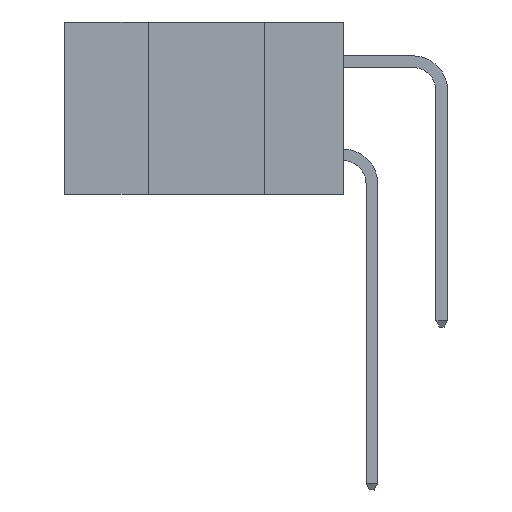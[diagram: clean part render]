
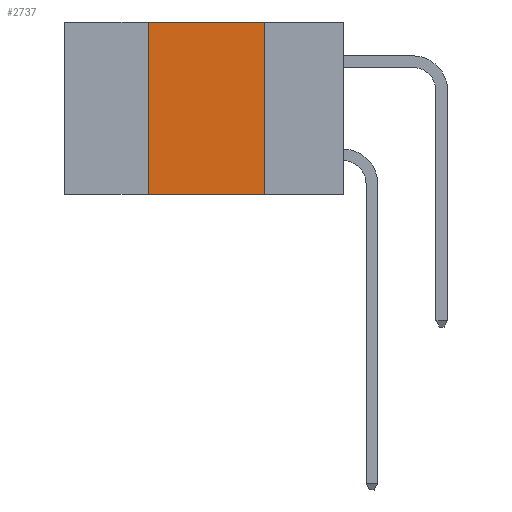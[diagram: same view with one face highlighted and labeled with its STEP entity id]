
A CAD part, left-side view. The second image highlights one B-rep face of the part: STEP entity #2737.
In plain terms, the highlighted planar face has unit normal (-1, 0, 0).
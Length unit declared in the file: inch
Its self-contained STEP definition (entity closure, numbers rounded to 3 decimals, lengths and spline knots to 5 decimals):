
#382 = DIRECTION ( 'NONE',  ( 0., -1., 0. ) ) ;
#444 = CARTESIAN_POINT ( 'NONE',  ( 0., 0.42, 0. ) ) ;
#821 = DIRECTION ( 'NONE',  ( 0., 0., 1. ) ) ;
#986 = CARTESIAN_POINT ( 'NONE',  ( 0., 0.42, -0.37 ) ) ;
#1899 = DIRECTION ( 'NONE',  ( 0., 0., -1. ) ) ;
#2342 = CARTESIAN_POINT ( 'NONE',  ( 0., 0.42, 0. ) ) ;
#2737 = ADVANCED_FACE ( 'NONE', ( #7547 ), #6748, .F. ) ;
#3230 = LINE ( 'NONE', #13689, #19517 ) ;
#4160 = CARTESIAN_POINT ( 'NONE',  ( 0., 0.6, 0. ) ) ;
#5080 = CARTESIAN_POINT ( 'NONE',  ( 0., 0.6, 0. ) ) ;
#5134 = VECTOR ( 'NONE', #821, 39.37008 ) ;
#5512 = LINE ( 'NONE', #9386, #15669 ) ;
#6301 = CARTESIAN_POINT ( 'NONE',  ( 0., 0.17, -0.37 ) ) ;
#6748 = PLANE ( 'NONE',  #14610 ) ;
#6756 = EDGE_CURVE ( 'NONE', #20666, #8106, #7747, .T. ) ;
#7547 = FACE_OUTER_BOUND ( 'NONE', #16509, .T. ) ;
#7600 = VECTOR ( 'NONE', #19569, 39.37008 ) ;
#7747 = LINE ( 'NONE', #2342, #5134 ) ;
#8106 = VERTEX_POINT ( 'NONE', #444 ) ;
#8134 = EDGE_CURVE ( 'NONE', #20666, #9131, #3230, .T. ) ;
#8920 = EDGE_CURVE ( 'NONE', #16882, #9131, #5512, .T. ) ;
#9131 = VERTEX_POINT ( 'NONE', #6301 ) ;
#9386 = CARTESIAN_POINT ( 'NONE',  ( 0., 0.17, 0. ) ) ;
#10846 = ORIENTED_EDGE ( 'NONE', *, *, #6756, .F. ) ;
#11188 = ORIENTED_EDGE ( 'NONE', *, *, #8134, .T. ) ;
#11877 = DIRECTION ( 'NONE',  ( 1., 0., 0. ) ) ;
#13689 = CARTESIAN_POINT ( 'NONE',  ( 0., 0.6, -0.37 ) ) ;
#14610 = AXIS2_PLACEMENT_3D ( 'NONE', #5080, #11877, #1899 ) ;
#14887 = ORIENTED_EDGE ( 'NONE', *, *, #8920, .F. ) ;
#15381 = EDGE_CURVE ( 'NONE', #8106, #16882, #16410, .T. ) ;
#15669 = VECTOR ( 'NONE', #19330, 39.37008 ) ;
#16410 = LINE ( 'NONE', #4160, #7600 ) ;
#16509 = EDGE_LOOP ( 'NONE', ( #14887, #19367, #10846, #11188 ) ) ;
#16882 = VERTEX_POINT ( 'NONE', #19993 ) ;
#19330 = DIRECTION ( 'NONE',  ( 0., 0., -1. ) ) ;
#19367 = ORIENTED_EDGE ( 'NONE', *, *, #15381, .F. ) ;
#19517 = VECTOR ( 'NONE', #382, 39.37008 ) ;
#19569 = DIRECTION ( 'NONE',  ( 0., -1., 0. ) ) ;
#19993 = CARTESIAN_POINT ( 'NONE',  ( 0., 0.17, 0. ) ) ;
#20666 = VERTEX_POINT ( 'NONE', #986 ) ;
